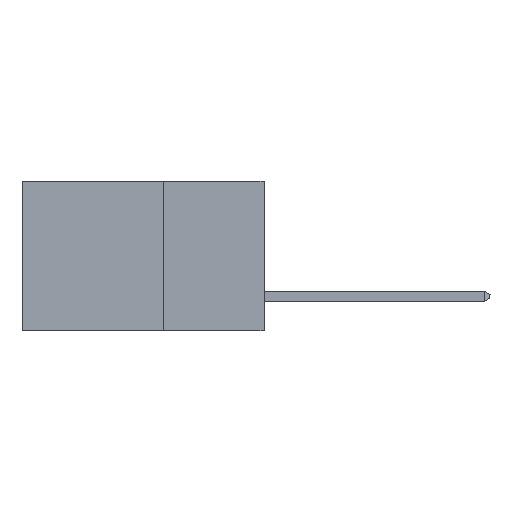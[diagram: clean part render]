
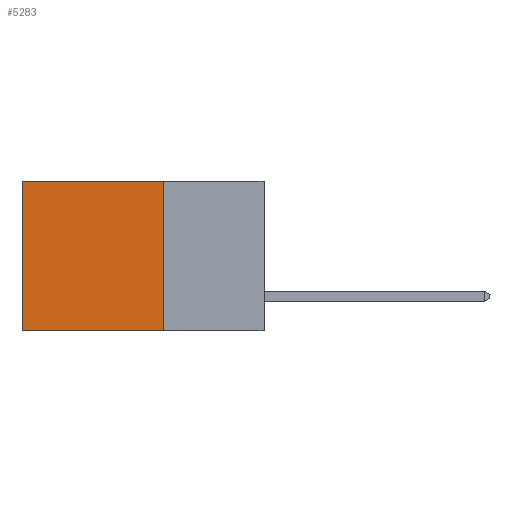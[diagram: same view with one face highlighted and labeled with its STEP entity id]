
A CAD part, left-side view. The second image highlights one B-rep face of the part: STEP entity #5283.
In plain terms, the highlighted planar face has unit normal (-1, 0, 0).
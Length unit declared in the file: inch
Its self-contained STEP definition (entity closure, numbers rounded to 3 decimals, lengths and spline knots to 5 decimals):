
#898 = VECTOR ( 'NONE', #12131, 39.37008 ) ;
#1009 = DIRECTION ( 'NONE',  ( 0., 0., -1. ) ) ;
#1070 = CARTESIAN_POINT ( 'NONE',  ( 0.2615, 0.6, -0.37 ) ) ;
#1279 = EDGE_CURVE ( 'NONE', #7968, #7424, #6901, .T. ) ;
#1884 = CARTESIAN_POINT ( 'NONE',  ( 0.2615, 0.6, 0. ) ) ;
#2069 = CARTESIAN_POINT ( 'NONE',  ( 0.2615, 0.25, -0.37 ) ) ;
#2257 = CARTESIAN_POINT ( 'NONE',  ( 0.2615, 0.25, -0.37 ) ) ;
#2327 = VECTOR ( 'NONE', #12071, 39.37008 ) ;
#3110 = PLANE ( 'NONE',  #5521 ) ;
#3247 = ORIENTED_EDGE ( 'NONE', *, *, #8802, .T. ) ;
#3677 = VECTOR ( 'NONE', #1009, 39.37008 ) ;
#4102 = EDGE_CURVE ( 'NONE', #7424, #7512, #6993, .T. ) ;
#4289 = CARTESIAN_POINT ( 'NONE',  ( 0.2615, 0.25, 0. ) ) ;
#5283 = ADVANCED_FACE ( 'NONE', ( #7198 ), #3110, .F. ) ;
#5521 = AXIS2_PLACEMENT_3D ( 'NONE', #2069, #12142, #6207 ) ;
#5990 = CARTESIAN_POINT ( 'NONE',  ( 0.2615, 0.25, -0.37 ) ) ;
#6001 = CARTESIAN_POINT ( 'NONE',  ( 0.2615, 0.6, -0.37 ) ) ;
#6048 = VECTOR ( 'NONE', #9733, 39.37008 ) ;
#6207 = DIRECTION ( 'NONE',  ( 0., 0., -1. ) ) ;
#6386 = EDGE_LOOP ( 'NONE', ( #8153, #7913, #8656, #3247 ) ) ;
#6901 = LINE ( 'NONE', #5990, #3677 ) ;
#6993 = LINE ( 'NONE', #2257, #2327 ) ;
#7010 = VERTEX_POINT ( 'NONE', #1884 ) ;
#7198 = FACE_OUTER_BOUND ( 'NONE', #6386, .T. ) ;
#7424 = VERTEX_POINT ( 'NONE', #12710 ) ;
#7512 = VERTEX_POINT ( 'NONE', #1070 ) ;
#7913 = ORIENTED_EDGE ( 'NONE', *, *, #4102, .F. ) ;
#7928 = CARTESIAN_POINT ( 'NONE',  ( 0.2615, 0.25, 0. ) ) ;
#7968 = VERTEX_POINT ( 'NONE', #7928 ) ;
#8153 = ORIENTED_EDGE ( 'NONE', *, *, #8708, .T. ) ;
#8656 = ORIENTED_EDGE ( 'NONE', *, *, #1279, .F. ) ;
#8708 = EDGE_CURVE ( 'NONE', #7010, #7512, #10836, .T. ) ;
#8802 = EDGE_CURVE ( 'NONE', #7968, #7010, #11220, .T. ) ;
#9733 = DIRECTION ( 'NONE',  ( 0., 0., -1. ) ) ;
#10836 = LINE ( 'NONE', #6001, #6048 ) ;
#11220 = LINE ( 'NONE', #4289, #898 ) ;
#12071 = DIRECTION ( 'NONE',  ( 0., 1., 0. ) ) ;
#12131 = DIRECTION ( 'NONE',  ( 0., 1., 0. ) ) ;
#12142 = DIRECTION ( 'NONE',  ( 1., 0., 0. ) ) ;
#12710 = CARTESIAN_POINT ( 'NONE',  ( 0.2615, 0.25, -0.37 ) ) ;
